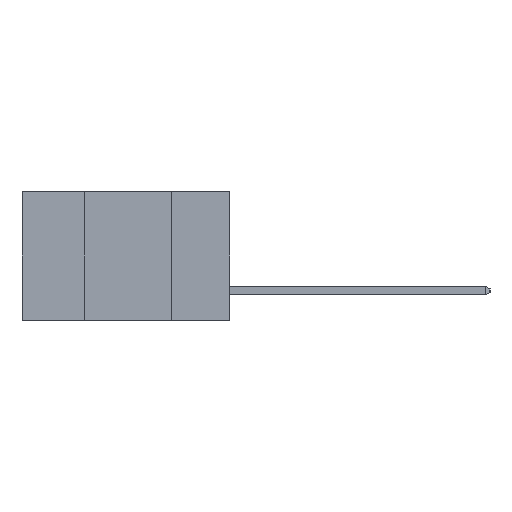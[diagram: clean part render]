
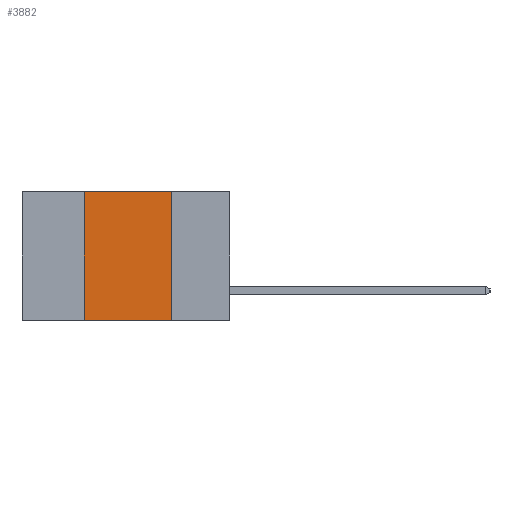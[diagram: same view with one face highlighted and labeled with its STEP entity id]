
A CAD part, left-side view. The second image highlights one B-rep face of the part: STEP entity #3882.
In plain terms, the highlighted planar face has unit normal (-1, 0, 0).
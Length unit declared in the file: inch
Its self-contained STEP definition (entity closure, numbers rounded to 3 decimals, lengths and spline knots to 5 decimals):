
#573 = VECTOR ( 'NONE', #18524, 39.37008 ) ;
#740 = CARTESIAN_POINT ( 'NONE',  ( 0., 0.42, 0. ) ) ;
#1614 = VERTEX_POINT ( 'NONE', #740 ) ;
#1864 = LINE ( 'NONE', #11442, #16361 ) ;
#3373 = CARTESIAN_POINT ( 'NONE',  ( 0., 0.42, -0.37 ) ) ;
#3882 = ADVANCED_FACE ( 'NONE', ( #13246 ), #5211, .F. ) ;
#4136 = DIRECTION ( 'NONE',  ( 0., 0., -1. ) ) ;
#4155 = DIRECTION ( 'NONE',  ( 0., -1., 0. ) ) ;
#4161 = DIRECTION ( 'NONE',  ( 1., 0., 0. ) ) ;
#4659 = CARTESIAN_POINT ( 'NONE',  ( 0., 0.6, 0. ) ) ;
#5211 = PLANE ( 'NONE',  #8269 ) ;
#5689 = CARTESIAN_POINT ( 'NONE',  ( 0., 0.42, -0.37 ) ) ;
#6500 = ORIENTED_EDGE ( 'NONE', *, *, #18081, .T. ) ;
#8269 = AXIS2_PLACEMENT_3D ( 'NONE', #4659, #4161, #4136 ) ;
#9015 = ORIENTED_EDGE ( 'NONE', *, *, #9463, .F. ) ;
#9463 = EDGE_CURVE ( 'NONE', #1614, #14625, #16487, .T. ) ;
#9623 = VERTEX_POINT ( 'NONE', #17284 ) ;
#11442 = CARTESIAN_POINT ( 'NONE',  ( 0., 0.17, -0.37 ) ) ;
#11554 = EDGE_LOOP ( 'NONE', ( #17659, #9015, #14576, #6500 ) ) ;
#13157 = CARTESIAN_POINT ( 'NONE',  ( 0., 0.6, -0.37 ) ) ;
#13246 = FACE_OUTER_BOUND ( 'NONE', #11554, .T. ) ;
#13433 = LINE ( 'NONE', #13157, #13896 ) ;
#13472 = LINE ( 'NONE', #3373, #13936 ) ;
#13884 = DIRECTION ( 'NONE',  ( 0., 0., 1. ) ) ;
#13896 = VECTOR ( 'NONE', #4155, 39.37008 ) ;
#13936 = VECTOR ( 'NONE', #13884, 39.37008 ) ;
#14404 = DIRECTION ( 'NONE',  ( 0., 0., -1. ) ) ;
#14576 = ORIENTED_EDGE ( 'NONE', *, *, #17307, .F. ) ;
#14625 = VERTEX_POINT ( 'NONE', #17264 ) ;
#16361 = VECTOR ( 'NONE', #14404, 39.37008 ) ;
#16487 = LINE ( 'NONE', #18715, #573 ) ;
#17264 = CARTESIAN_POINT ( 'NONE',  ( 0., 0.17, 0. ) ) ;
#17284 = CARTESIAN_POINT ( 'NONE',  ( 0., 0.17, -0.37 ) ) ;
#17307 = EDGE_CURVE ( 'NONE', #18158, #1614, #13472, .T. ) ;
#17659 = ORIENTED_EDGE ( 'NONE', *, *, #19072, .F. ) ;
#18081 = EDGE_CURVE ( 'NONE', #18158, #9623, #13433, .T. ) ;
#18158 = VERTEX_POINT ( 'NONE', #5689 ) ;
#18524 = DIRECTION ( 'NONE',  ( 0., -1., 0. ) ) ;
#18715 = CARTESIAN_POINT ( 'NONE',  ( 0., 0.6, 0. ) ) ;
#19072 = EDGE_CURVE ( 'NONE', #14625, #9623, #1864, .T. ) ;
